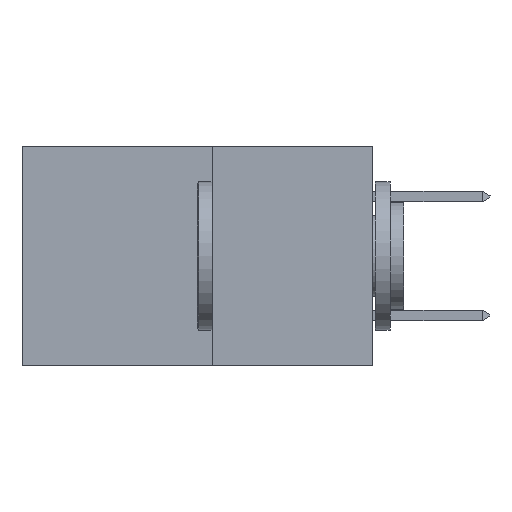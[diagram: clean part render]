
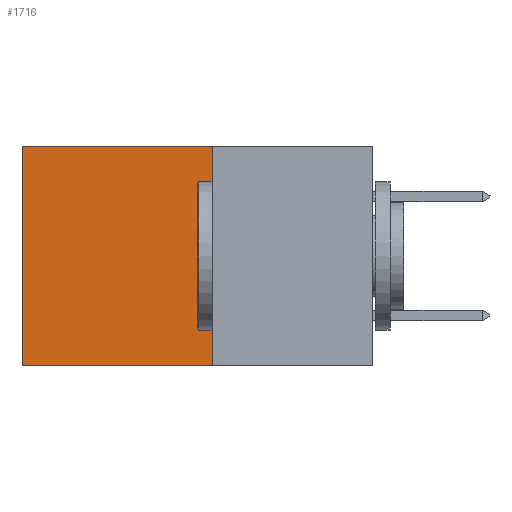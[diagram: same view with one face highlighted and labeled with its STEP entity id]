
A CAD part, left-side view. The second image highlights one B-rep face of the part: STEP entity #1716.
In plain terms, the highlighted planar face has unit normal (-1, 0, 0).
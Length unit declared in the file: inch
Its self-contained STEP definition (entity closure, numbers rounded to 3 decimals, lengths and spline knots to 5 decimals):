
#1716 = ADVANCED_FACE ( 'NONE', ( #34604 ), #12933, .F. ) ;
#2608 = AXIS2_PLACEMENT_3D ( 'NONE', #12699, #6227, #10271 ) ;
#2762 = VECTOR ( 'NONE', #25369, 39.37008 ) ;
#3835 = CARTESIAN_POINT ( 'NONE',  ( 0.277, 0.27, -0.37 ) ) ;
#4141 = EDGE_CURVE ( 'NONE', #20332, #9348, #12488, .T. ) ;
#4675 = DIRECTION ( 'NONE',  ( 0., 1., 0. ) ) ;
#6227 = DIRECTION ( 'NONE',  ( 1., 0., 0. ) ) ;
#7250 = ORIENTED_EDGE ( 'NONE', *, *, #15625, .T. ) ;
#9324 = EDGE_CURVE ( 'NONE', #25407, #22753, #14729, .T. ) ;
#9348 = VERTEX_POINT ( 'NONE', #27766 ) ;
#10271 = DIRECTION ( 'NONE',  ( 0., 0., -1. ) ) ;
#11119 = CARTESIAN_POINT ( 'NONE',  ( 0.277, 0.27, -0.37 ) ) ;
#12488 = LINE ( 'NONE', #28866, #33177 ) ;
#12699 = CARTESIAN_POINT ( 'NONE',  ( 0.277, 0.27, -0.37 ) ) ;
#12919 = ORIENTED_EDGE ( 'NONE', *, *, #9324, .F. ) ;
#12933 = PLANE ( 'NONE',  #2608 ) ;
#14729 = LINE ( 'NONE', #24953, #34523 ) ;
#15345 = EDGE_LOOP ( 'NONE', ( #18895, #25074, #12919, #7250 ) ) ;
#15625 = EDGE_CURVE ( 'NONE', #25407, #20332, #33492, .T. ) ;
#18137 = CARTESIAN_POINT ( 'NONE',  ( 0.277, 0.27, 0. ) ) ;
#18895 = ORIENTED_EDGE ( 'NONE', *, *, #4141, .T. ) ;
#19556 = DIRECTION ( 'NONE',  ( 0., 0., -1. ) ) ;
#20032 = VECTOR ( 'NONE', #4675, 39.37008 ) ;
#20332 = VERTEX_POINT ( 'NONE', #20957 ) ;
#20837 = CARTESIAN_POINT ( 'NONE',  ( 0.277, 0.27, 0. ) ) ;
#20957 = CARTESIAN_POINT ( 'NONE',  ( 0.277, 0.59, 0. ) ) ;
#22753 = VERTEX_POINT ( 'NONE', #11119 ) ;
#23425 = LINE ( 'NONE', #3835, #2762 ) ;
#24516 = EDGE_CURVE ( 'NONE', #22753, #9348, #23425, .T. ) ;
#24953 = CARTESIAN_POINT ( 'NONE',  ( 0.277, 0.27, -0.37 ) ) ;
#25074 = ORIENTED_EDGE ( 'NONE', *, *, #24516, .F. ) ;
#25369 = DIRECTION ( 'NONE',  ( 0., 1., 0. ) ) ;
#25407 = VERTEX_POINT ( 'NONE', #18137 ) ;
#27766 = CARTESIAN_POINT ( 'NONE',  ( 0.277, 0.59, -0.37 ) ) ;
#28866 = CARTESIAN_POINT ( 'NONE',  ( 0.277, 0.59, -0.37 ) ) ;
#29507 = DIRECTION ( 'NONE',  ( 0., 0., -1. ) ) ;
#33177 = VECTOR ( 'NONE', #29507, 39.37008 ) ;
#33492 = LINE ( 'NONE', #20837, #20032 ) ;
#34523 = VECTOR ( 'NONE', #19556, 39.37008 ) ;
#34604 = FACE_OUTER_BOUND ( 'NONE', #15345, .T. ) ;
